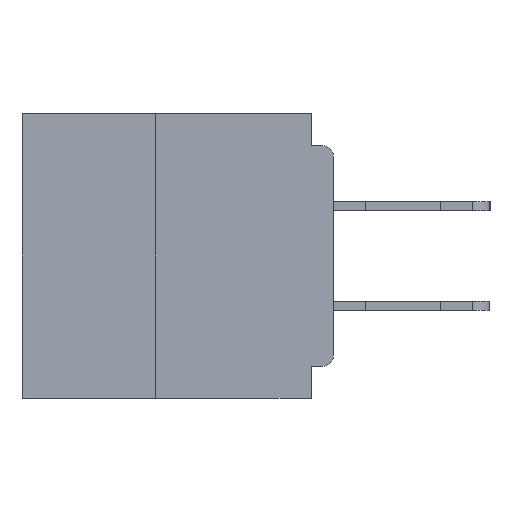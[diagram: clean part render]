
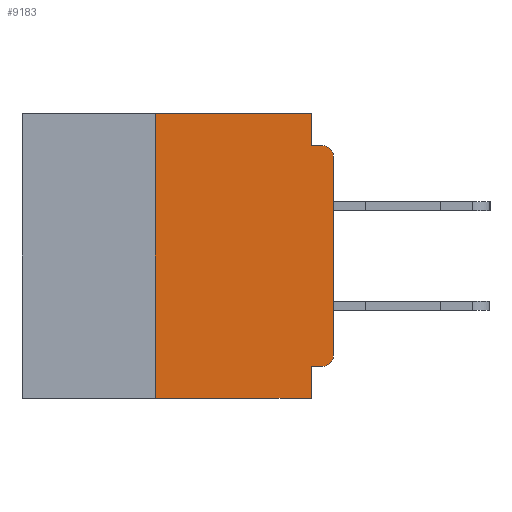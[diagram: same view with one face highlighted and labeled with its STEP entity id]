
A CAD part, left-side view. The second image highlights one B-rep face of the part: STEP entity #9183.
In plain terms, the highlighted planar face has unit normal (-1, 0, 0).
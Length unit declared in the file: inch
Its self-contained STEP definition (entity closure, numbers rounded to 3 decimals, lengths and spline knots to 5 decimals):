
#592 = VERTEX_POINT ( 'NONE', #1684 ) ;
#898 = DIRECTION ( 'NONE',  ( 0., 0., -1. ) ) ;
#1322 = VECTOR ( 'NONE', #15562, 39.37008 ) ;
#1594 = VECTOR ( 'NONE', #45312, 39.37008 ) ;
#1684 = CARTESIAN_POINT ( 'NONE',  ( 0., 0.25, -0.4 ) ) ;
#1809 = ORIENTED_EDGE ( 'NONE', *, *, #26021, .T. ) ;
#1883 = EDGE_CURVE ( 'NONE', #592, #31037, #9894, .T. ) ;
#2127 = ORIENTED_EDGE ( 'NONE', *, *, #44385, .T. ) ;
#2322 = ORIENTED_EDGE ( 'NONE', *, *, #14808, .F. ) ;
#2412 = ORIENTED_EDGE ( 'NONE', *, *, #32059, .F. ) ;
#3190 = ORIENTED_EDGE ( 'NONE', *, *, #30361, .F. ) ;
#3298 = ORIENTED_EDGE ( 'NONE', *, *, #43755, .F. ) ;
#4151 = ORIENTED_EDGE ( 'NONE', *, *, #1883, .T. ) ;
#5166 = ORIENTED_EDGE ( 'NONE', *, *, #28289, .F. ) ;
#5594 = CARTESIAN_POINT ( 'NONE',  ( 0., 0.031, -0.045 ) ) ;
#5925 = DIRECTION ( 'NONE',  ( 0., 0., 1. ) ) ;
#7042 = DIRECTION ( 'NONE',  ( 0., 0., -1. ) ) ;
#7366 = EDGE_CURVE ( 'NONE', #12336, #21725, #46106, .T. ) ;
#7393 = VERTEX_POINT ( 'NONE', #41623 ) ;
#8507 = CARTESIAN_POINT ( 'NONE',  ( 0., 0., -0.355 ) ) ;
#8777 = ORIENTED_EDGE ( 'NONE', *, *, #10444, .F. ) ;
#9081 = LINE ( 'NONE', #20462, #17664 ) ;
#9183 = ADVANCED_FACE ( 'NONE', ( #39011 ), #44941, .F. ) ;
#9247 = ORIENTED_EDGE ( 'NONE', *, *, #7366, .T. ) ;
#9894 = LINE ( 'NONE', #29260, #1322 ) ;
#10444 = EDGE_CURVE ( 'NONE', #12336, #47115, #22225, .T. ) ;
#10483 = CARTESIAN_POINT ( 'NONE',  ( 0., 0.437, 0. ) ) ;
#12336 = VERTEX_POINT ( 'NONE', #27148 ) ;
#13906 = AXIS2_PLACEMENT_3D ( 'NONE', #41087, #22841, #898 ) ;
#14808 = EDGE_CURVE ( 'NONE', #36750, #7393, #31771, .T. ) ;
#15562 = DIRECTION ( 'NONE',  ( 0., -1., 0. ) ) ;
#15670 = VERTEX_POINT ( 'NONE', #26317 ) ;
#15732 = VECTOR ( 'NONE', #39937, 39.37008 ) ;
#15959 = CARTESIAN_POINT ( 'NONE',  ( 0., 0.031, -0.4 ) ) ;
#17664 = VECTOR ( 'NONE', #5925, 39.37008 ) ;
#18124 = CARTESIAN_POINT ( 'NONE',  ( 0., 0.031, -0.4 ) ) ;
#18134 = VERTEX_POINT ( 'NONE', #37948 ) ;
#18494 = VECTOR ( 'NONE', #7042, 39.37008 ) ;
#19359 = CARTESIAN_POINT ( 'NONE',  ( 0., 0.015, -0.34 ) ) ;
#19673 = DIRECTION ( 'NONE',  ( -1., 0., 0. ) ) ;
#20462 = CARTESIAN_POINT ( 'NONE',  ( 0., 0., 0. ) ) ;
#21498 = EDGE_LOOP ( 'NONE', ( #1809, #2127, #2322, #2412, #3190, #3298, #4151, #5166, #8777, #9247 ) ) ;
#21580 = CARTESIAN_POINT ( 'NONE',  ( 0., 0.031, 0. ) ) ;
#21675 = DIRECTION ( 'NONE',  ( 0., -1., 0. ) ) ;
#21725 = VERTEX_POINT ( 'NONE', #39597 ) ;
#22225 = LINE ( 'NONE', #8507, #1594 ) ;
#22582 = VECTOR ( 'NONE', #45410, 39.37008 ) ;
#22841 = DIRECTION ( 'NONE',  ( 1., 0., 0. ) ) ;
#23061 = DIRECTION ( 'NONE',  ( 0., 0., -1. ) ) ;
#23368 = AXIS2_PLACEMENT_3D ( 'NONE', #41792, #19673, #45463 ) ;
#26021 = EDGE_CURVE ( 'NONE', #21725, #15670, #9081, .T. ) ;
#26317 = CARTESIAN_POINT ( 'NONE',  ( 0., 0., -0.06 ) ) ;
#27148 = CARTESIAN_POINT ( 'NONE',  ( 0., 0.015, -0.355 ) ) ;
#28289 = EDGE_CURVE ( 'NONE', #47115, #31037, #33615, .T. ) ;
#28297 = LINE ( 'NONE', #21580, #18494 ) ;
#29126 = LINE ( 'NONE', #38147, #47535 ) ;
#29260 = CARTESIAN_POINT ( 'NONE',  ( 0., 0.437, -0.4 ) ) ;
#30361 = EDGE_CURVE ( 'NONE', #18134, #36628, #37672, .T. ) ;
#30919 = CARTESIAN_POINT ( 'NONE',  ( 0., 0.031, -0.355 ) ) ;
#31037 = VERTEX_POINT ( 'NONE', #18124 ) ;
#31771 = LINE ( 'NONE', #40051, #39215 ) ;
#32059 = EDGE_CURVE ( 'NONE', #36628, #36750, #28297, .T. ) ;
#33615 = LINE ( 'NONE', #15959, #22582 ) ;
#34374 = CARTESIAN_POINT ( 'NONE',  ( 0., 0.031, 0. ) ) ;
#36628 = VERTEX_POINT ( 'NONE', #34374 ) ;
#36750 = VERTEX_POINT ( 'NONE', #5594 ) ;
#37655 = AXIS2_PLACEMENT_3D ( 'NONE', #19359, #45149, #23061 ) ;
#37672 = LINE ( 'NONE', #10483, #15732 ) ;
#37948 = CARTESIAN_POINT ( 'NONE',  ( 0., 0.25, 0. ) ) ;
#38147 = CARTESIAN_POINT ( 'NONE',  ( 0., 0.25, -0.4 ) ) ;
#39011 = FACE_OUTER_BOUND ( 'NONE', #21498, .T. ) ;
#39215 = VECTOR ( 'NONE', #21675, 39.37008 ) ;
#39597 = CARTESIAN_POINT ( 'NONE',  ( 0., 0., -0.34 ) ) ;
#39937 = DIRECTION ( 'NONE',  ( 0., -1., 0. ) ) ;
#40051 = CARTESIAN_POINT ( 'NONE',  ( 0., 0., -0.045 ) ) ;
#41087 = CARTESIAN_POINT ( 'NONE',  ( 0., 0.437, 0. ) ) ;
#41623 = CARTESIAN_POINT ( 'NONE',  ( 0., 0.015, -0.045 ) ) ;
#41770 = CIRCLE ( 'NONE', #23368, 0.015 ) ;
#41792 = CARTESIAN_POINT ( 'NONE',  ( 0., 0.015, -0.06 ) ) ;
#41841 = DIRECTION ( 'NONE',  ( 0., 0., 1. ) ) ;
#43755 = EDGE_CURVE ( 'NONE', #592, #18134, #29126, .T. ) ;
#44385 = EDGE_CURVE ( 'NONE', #15670, #7393, #41770, .T. ) ;
#44941 = PLANE ( 'NONE',  #13906 ) ;
#45149 = DIRECTION ( 'NONE',  ( -1., 0., 0. ) ) ;
#45312 = DIRECTION ( 'NONE',  ( 0., 1., 0. ) ) ;
#45410 = DIRECTION ( 'NONE',  ( 0., 0., -1. ) ) ;
#45463 = DIRECTION ( 'NONE',  ( 0., 0., -1. ) ) ;
#46106 = CIRCLE ( 'NONE', #37655, 0.015 ) ;
#47115 = VERTEX_POINT ( 'NONE', #30919 ) ;
#47535 = VECTOR ( 'NONE', #41841, 39.37008 ) ;
